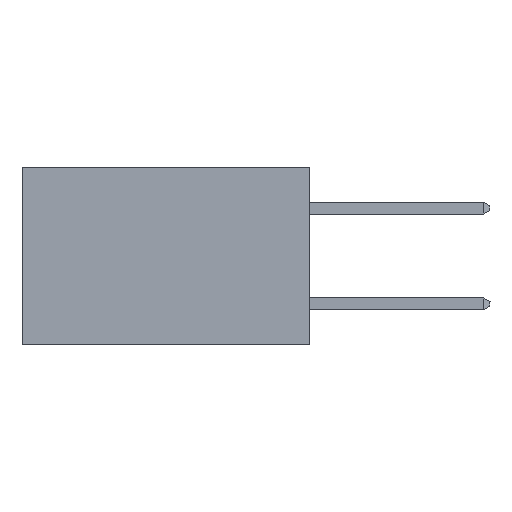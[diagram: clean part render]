
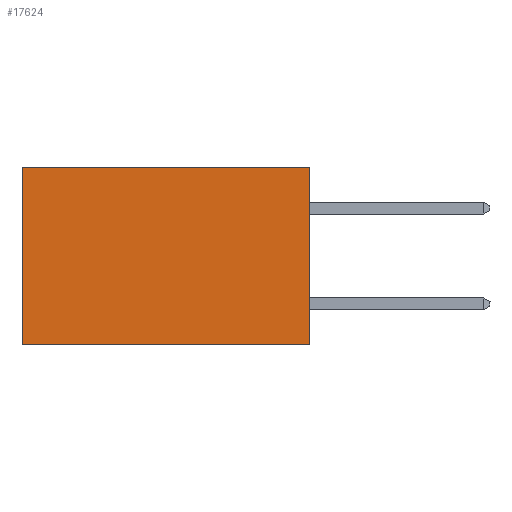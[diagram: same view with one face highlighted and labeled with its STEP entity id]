
A CAD part, left-side view. The second image highlights one B-rep face of the part: STEP entity #17624.
In plain terms, the highlighted planar face has unit normal (-1, 0, 0).
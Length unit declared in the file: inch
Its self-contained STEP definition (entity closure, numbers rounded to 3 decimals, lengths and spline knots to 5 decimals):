
#2383 = DIRECTION ( 'NONE',  ( 0., 0., -1. ) ) ;
#5417 = VERTEX_POINT ( 'NONE', #35165 ) ;
#6284 = CARTESIAN_POINT ( 'NONE',  ( 0.2875, 0.6, 0. ) ) ;
#7781 = CARTESIAN_POINT ( 'NONE',  ( 0.2875, 0.6, -0.37 ) ) ;
#9645 = VECTOR ( 'NONE', #2383, 39.37008 ) ;
#12384 = VERTEX_POINT ( 'NONE', #30592 ) ;
#12486 = DIRECTION ( 'NONE',  ( 0., 0., -1. ) ) ;
#14208 = FACE_OUTER_BOUND ( 'NONE', #33774, .T. ) ;
#14707 = EDGE_CURVE ( 'NONE', #35339, #24020, #40276, .T. ) ;
#14970 = AXIS2_PLACEMENT_3D ( 'NONE', #37768, #24787, #31289 ) ;
#15680 = EDGE_CURVE ( 'NONE', #12384, #24020, #39187, .T. ) ;
#16939 = EDGE_CURVE ( 'NONE', #5417, #12384, #40598, .T. ) ;
#17624 = ADVANCED_FACE ( 'NONE', ( #14208 ), #34258, .F. ) ;
#17771 = ORIENTED_EDGE ( 'NONE', *, *, #37385, .F. ) ;
#19074 = CARTESIAN_POINT ( 'NONE',  ( 0.2875, 0., -0.37 ) ) ;
#24020 = VERTEX_POINT ( 'NONE', #7781 ) ;
#24787 = DIRECTION ( 'NONE',  ( 1., 0., 0. ) ) ;
#25531 = VECTOR ( 'NONE', #12486, 39.37008 ) ;
#26910 = ORIENTED_EDGE ( 'NONE', *, *, #15680, .T. ) ;
#27370 = LINE ( 'NONE', #28165, #9645 ) ;
#27992 = VECTOR ( 'NONE', #36597, 39.37008 ) ;
#28165 = CARTESIAN_POINT ( 'NONE',  ( 0.2875, 0., 0. ) ) ;
#29962 = DIRECTION ( 'NONE',  ( 0., 1., 0. ) ) ;
#30045 = ORIENTED_EDGE ( 'NONE', *, *, #14707, .F. ) ;
#30592 = CARTESIAN_POINT ( 'NONE',  ( 0.2875, 0.6, 0. ) ) ;
#31289 = DIRECTION ( 'NONE',  ( 0., 0., -1. ) ) ;
#33774 = EDGE_LOOP ( 'NONE', ( #26910, #30045, #17771, #37476 ) ) ;
#34258 = PLANE ( 'NONE',  #14970 ) ;
#35165 = CARTESIAN_POINT ( 'NONE',  ( 0.2875, 0., 0. ) ) ;
#35339 = VERTEX_POINT ( 'NONE', #19074 ) ;
#36020 = CARTESIAN_POINT ( 'NONE',  ( 0.2875, 0., -0.37 ) ) ;
#36449 = CARTESIAN_POINT ( 'NONE',  ( 0.2875, 0., 0. ) ) ;
#36597 = DIRECTION ( 'NONE',  ( 0., 1., 0. ) ) ;
#37385 = EDGE_CURVE ( 'NONE', #5417, #35339, #27370, .T. ) ;
#37476 = ORIENTED_EDGE ( 'NONE', *, *, #16939, .T. ) ;
#37768 = CARTESIAN_POINT ( 'NONE',  ( 0.2875, 0., 0. ) ) ;
#38245 = VECTOR ( 'NONE', #29962, 39.37008 ) ;
#39187 = LINE ( 'NONE', #6284, #25531 ) ;
#40276 = LINE ( 'NONE', #36020, #38245 ) ;
#40598 = LINE ( 'NONE', #36449, #27992 ) ;
